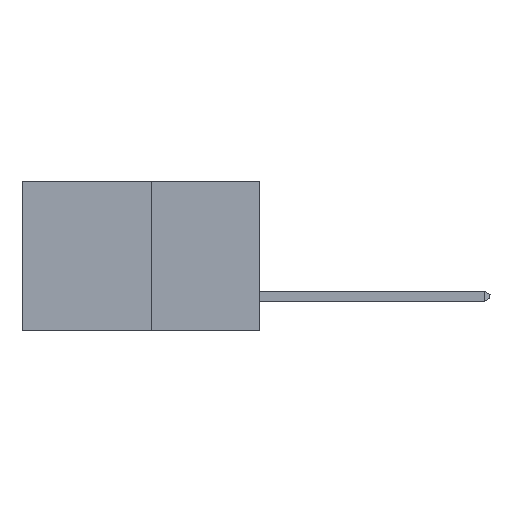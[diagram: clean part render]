
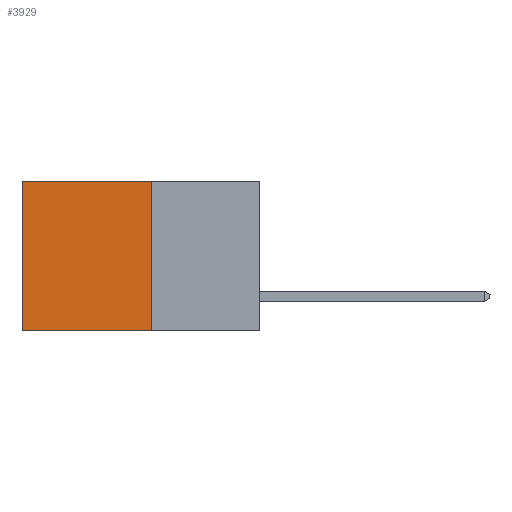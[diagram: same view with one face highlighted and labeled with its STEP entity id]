
A CAD part, left-side view. The second image highlights one B-rep face of the part: STEP entity #3929.
In plain terms, the highlighted planar face has unit normal (-1, 0, 0).
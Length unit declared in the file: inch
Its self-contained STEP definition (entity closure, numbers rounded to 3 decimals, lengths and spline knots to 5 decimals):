
#534 = VERTEX_POINT ( 'NONE', #13361 ) ;
#936 = VERTEX_POINT ( 'NONE', #19378 ) ;
#1695 = FACE_OUTER_BOUND ( 'NONE', #8354, .T. ) ;
#2691 = AXIS2_PLACEMENT_3D ( 'NONE', #4601, #4492, #4471 ) ;
#3826 = LINE ( 'NONE', #11395, #19749 ) ;
#3929 = ADVANCED_FACE ( 'NONE', ( #1695 ), #4678, .F. ) ;
#4108 = CARTESIAN_POINT ( 'NONE',  ( 0.277, 0.27, -0.37 ) ) ;
#4471 = DIRECTION ( 'NONE',  ( 0., 0., -1. ) ) ;
#4492 = DIRECTION ( 'NONE',  ( 1., 0., 0. ) ) ;
#4601 = CARTESIAN_POINT ( 'NONE',  ( 0.277, 0.27, -0.37 ) ) ;
#4678 = PLANE ( 'NONE',  #2691 ) ;
#4804 = LINE ( 'NONE', #12935, #16681 ) ;
#5003 = ORIENTED_EDGE ( 'NONE', *, *, #9450, .F. ) ;
#5136 = VERTEX_POINT ( 'NONE', #11884 ) ;
#5233 = DIRECTION ( 'NONE',  ( 0., 0., -1. ) ) ;
#5342 = VECTOR ( 'NONE', #16103, 39.37008 ) ;
#5806 = LINE ( 'NONE', #6726, #5342 ) ;
#5824 = CARTESIAN_POINT ( 'NONE',  ( 0.277, 0.27, -0.37 ) ) ;
#6084 = LINE ( 'NONE', #5824, #13905 ) ;
#6726 = CARTESIAN_POINT ( 'NONE',  ( 0.277, 0.59, -0.37 ) ) ;
#8354 = EDGE_LOOP ( 'NONE', ( #9767, #5003, #9697, #16907 ) ) ;
#9450 = EDGE_CURVE ( 'NONE', #18023, #5136, #6084, .T. ) ;
#9697 = ORIENTED_EDGE ( 'NONE', *, *, #11235, .F. ) ;
#9767 = ORIENTED_EDGE ( 'NONE', *, *, #10544, .T. ) ;
#10544 = EDGE_CURVE ( 'NONE', #936, #5136, #5806, .T. ) ;
#11201 = EDGE_CURVE ( 'NONE', #534, #936, #4804, .T. ) ;
#11235 = EDGE_CURVE ( 'NONE', #534, #18023, #3826, .T. ) ;
#11395 = CARTESIAN_POINT ( 'NONE',  ( 0.277, 0.27, -0.37 ) ) ;
#11884 = CARTESIAN_POINT ( 'NONE',  ( 0.277, 0.59, -0.37 ) ) ;
#12935 = CARTESIAN_POINT ( 'NONE',  ( 0.277, 0.27, 0. ) ) ;
#13361 = CARTESIAN_POINT ( 'NONE',  ( 0.277, 0.27, 0. ) ) ;
#13905 = VECTOR ( 'NONE', #18198, 39.37008 ) ;
#14497 = DIRECTION ( 'NONE',  ( 0., 1., 0. ) ) ;
#16103 = DIRECTION ( 'NONE',  ( 0., 0., -1. ) ) ;
#16681 = VECTOR ( 'NONE', #14497, 39.37008 ) ;
#16907 = ORIENTED_EDGE ( 'NONE', *, *, #11201, .T. ) ;
#18023 = VERTEX_POINT ( 'NONE', #4108 ) ;
#18198 = DIRECTION ( 'NONE',  ( 0., 1., 0. ) ) ;
#19378 = CARTESIAN_POINT ( 'NONE',  ( 0.277, 0.59, 0. ) ) ;
#19749 = VECTOR ( 'NONE', #5233, 39.37008 ) ;
